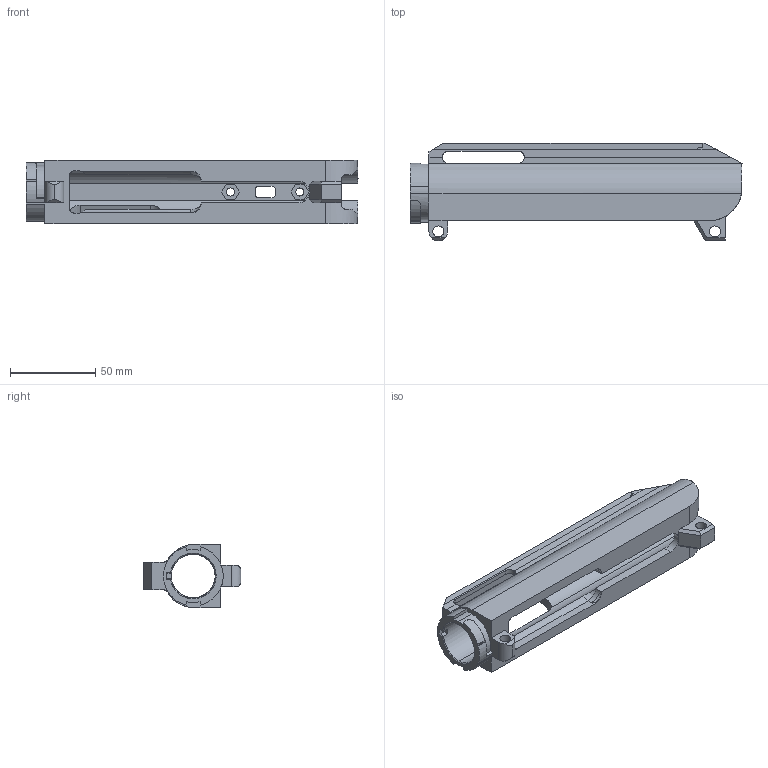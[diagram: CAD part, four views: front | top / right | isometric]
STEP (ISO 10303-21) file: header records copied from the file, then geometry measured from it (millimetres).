
FILE_DESCRIPTION (( 'STEP AP214' ), '1' );
FILE_NAME ('Upper.step', '2019-12-18T03:09:08', ( '' ), ( '' ), 'SwSTEP 2.0', 'SolidWorks 2019', '' );
FILE_SCHEMA (( 'AUTOMOTIVE_DESIGN' ));
Length unit declared in the file: millimetre
Products named in the file (1): Upper
Bounding box: 194.41 x 57.13 x 37.15 mm (x, y, z)
Volume: 101670.9 mm3; surface area: 53074.7 mm2
Topology: 2 solids, 8 shells, 242 faces, 690 edges, 458 vertices
Faces by surface type: plane 135, cylinder 83, bspline 13, torus 6, cone 3, sphere 2
Entity records: 9512 total; most frequent: CARTESIAN_POINT 3251, ORIENTED_EDGE 1380, DIRECTION 1201, EDGE_CURVE 690, VERTEX_POINT 458, VECTOR 417, LINE 417, AXIS2_PLACEMENT_3D 392
